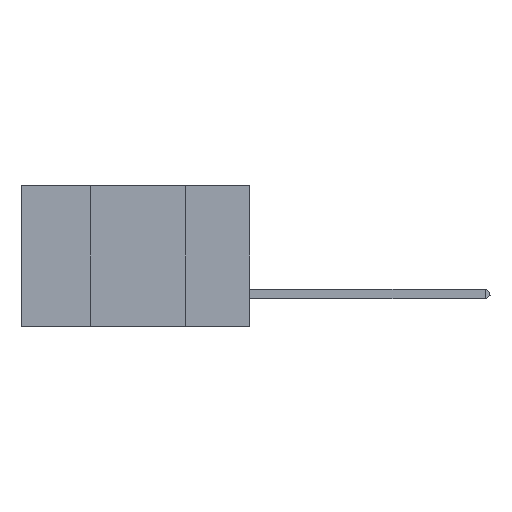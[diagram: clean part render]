
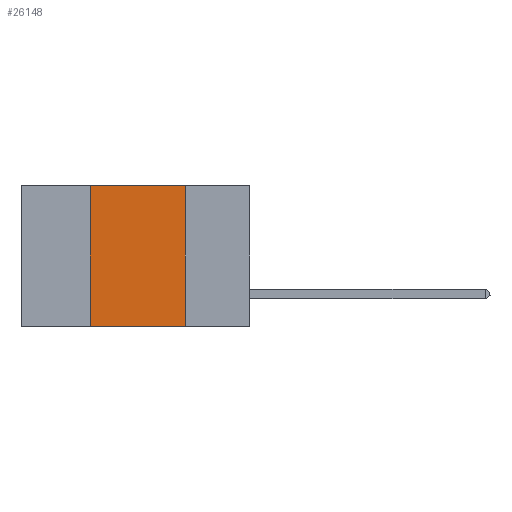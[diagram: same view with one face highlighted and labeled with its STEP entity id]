
A CAD part, left-side view. The second image highlights one B-rep face of the part: STEP entity #26148.
In plain terms, the highlighted planar face has unit normal (-1, 0, 0).
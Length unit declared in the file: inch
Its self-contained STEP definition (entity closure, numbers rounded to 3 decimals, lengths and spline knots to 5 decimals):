
#118 = LINE ( 'NONE', #15908, #16916 ) ;
#963 = CARTESIAN_POINT ( 'NONE',  ( 0., 0.42, -0.37 ) ) ;
#1707 = VERTEX_POINT ( 'NONE', #17990 ) ;
#2278 = PLANE ( 'NONE',  #24789 ) ;
#2636 = CARTESIAN_POINT ( 'NONE',  ( 0., 0.6, 0. ) ) ;
#2747 = CARTESIAN_POINT ( 'NONE',  ( 0., 0.42, 0. ) ) ;
#3559 = DIRECTION ( 'NONE',  ( 0., 0., -1. ) ) ;
#4318 = VERTEX_POINT ( 'NONE', #963 ) ;
#6767 = CARTESIAN_POINT ( 'NONE',  ( 0., 0.17, 0. ) ) ;
#7269 = EDGE_CURVE ( 'NONE', #1707, #8569, #25459, .T. ) ;
#7679 = ORIENTED_EDGE ( 'NONE', *, *, #25331, .T. ) ;
#8166 = VECTOR ( 'NONE', #25811, 39.37008 ) ;
#8569 = VERTEX_POINT ( 'NONE', #6767 ) ;
#10081 = CARTESIAN_POINT ( 'NONE',  ( 0., 0.17, -0.37 ) ) ;
#13320 = DIRECTION ( 'NONE',  ( 0., 0., -1. ) ) ;
#13599 = DIRECTION ( 'NONE',  ( 0., 0., 1. ) ) ;
#14592 = EDGE_CURVE ( 'NONE', #4318, #1707, #26605, .T. ) ;
#15029 = VECTOR ( 'NONE', #3559, 39.37008 ) ;
#15105 = CARTESIAN_POINT ( 'NONE',  ( 0., 0.6, 0. ) ) ;
#15908 = CARTESIAN_POINT ( 'NONE',  ( 0., 0.6, -0.37 ) ) ;
#15957 = FACE_OUTER_BOUND ( 'NONE', #30214, .T. ) ;
#16401 = ORIENTED_EDGE ( 'NONE', *, *, #7269, .F. ) ;
#16916 = VECTOR ( 'NONE', #18368, 39.37008 ) ;
#17990 = CARTESIAN_POINT ( 'NONE',  ( 0., 0.42, 0. ) ) ;
#18368 = DIRECTION ( 'NONE',  ( 0., -1., 0. ) ) ;
#18880 = ORIENTED_EDGE ( 'NONE', *, *, #24219, .F. ) ;
#19870 = LINE ( 'NONE', #24784, #15029 ) ;
#22875 = ORIENTED_EDGE ( 'NONE', *, *, #14592, .F. ) ;
#24219 = EDGE_CURVE ( 'NONE', #8569, #28387, #19870, .T. ) ;
#24784 = CARTESIAN_POINT ( 'NONE',  ( 0., 0.17, 0. ) ) ;
#24789 = AXIS2_PLACEMENT_3D ( 'NONE', #2636, #26315, #13320 ) ;
#25331 = EDGE_CURVE ( 'NONE', #4318, #28387, #118, .T. ) ;
#25459 = LINE ( 'NONE', #15105, #8166 ) ;
#25811 = DIRECTION ( 'NONE',  ( 0., -1., 0. ) ) ;
#26148 = ADVANCED_FACE ( 'NONE', ( #15957 ), #2278, .F. ) ;
#26315 = DIRECTION ( 'NONE',  ( 1., 0., 0. ) ) ;
#26605 = LINE ( 'NONE', #2747, #27073 ) ;
#27073 = VECTOR ( 'NONE', #13599, 39.37008 ) ;
#28387 = VERTEX_POINT ( 'NONE', #10081 ) ;
#30214 = EDGE_LOOP ( 'NONE', ( #18880, #16401, #22875, #7679 ) ) ;
